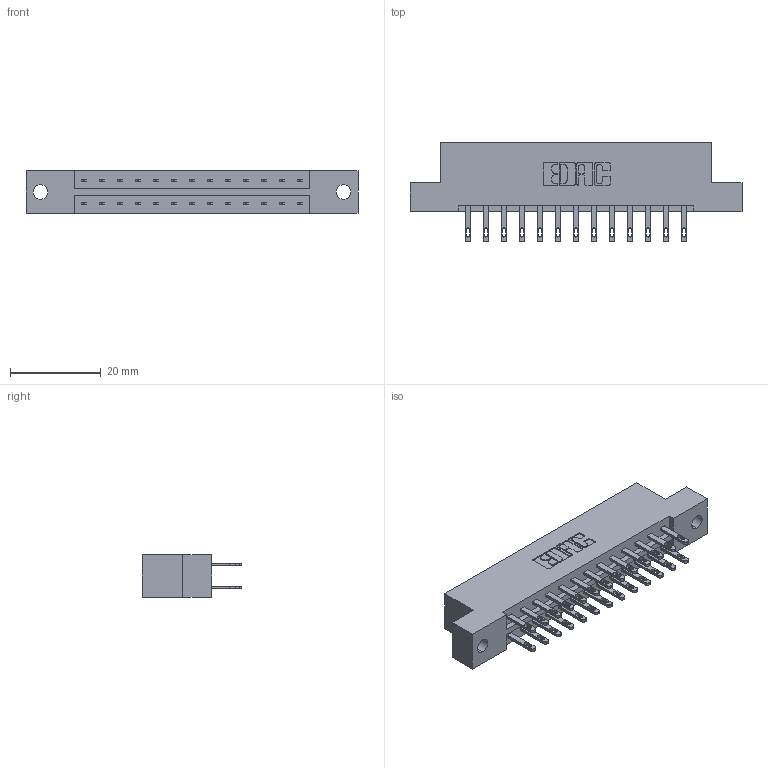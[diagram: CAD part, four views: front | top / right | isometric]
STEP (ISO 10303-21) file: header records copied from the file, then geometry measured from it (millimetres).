
FILE_DESCRIPTION (( 'STEP AP203' ), '1' );
FILE_NAME ('833-026-500-202.STEP', '2020-06-02T00:26:40', ( '' ), ( '' ), 'SwSTEP 2.0', 'SolidWorks 2020', '' );
FILE_SCHEMA (( 'CONFIG_CONTROL_DESIGN' ));
Length unit declared in the file: inch
Products named in the file (3): 345-292-001_345-293-100; 833 Part_Flush - .128 Dia; 833-026-500-202
Assembly tree (27 placements, depth 2):
  833-026-500-202
    833 Part_Flush - .128 Dia
    345-292-001_345-293-100  x26
Bounding box: 73.05 x 21.85 x 9.4 mm (x, y, z)
Volume: 7229.6 mm3; surface area: 8248.3 mm2
Topology: 27 solids, 27 shells, 1362 faces, 4133 edges, 2754 vertices
Faces by surface type: plane 850, cylinder 512
Entity records: 12047 total; most frequent: CARTESIAN_POINT 2030, ORIENTED_EDGE 1966, DIRECTION 1787, EDGE_CURVE 983, LINE 851, VECTOR 851, VERTEX_POINT 654, AXIS2_PLACEMENT_3D 468
